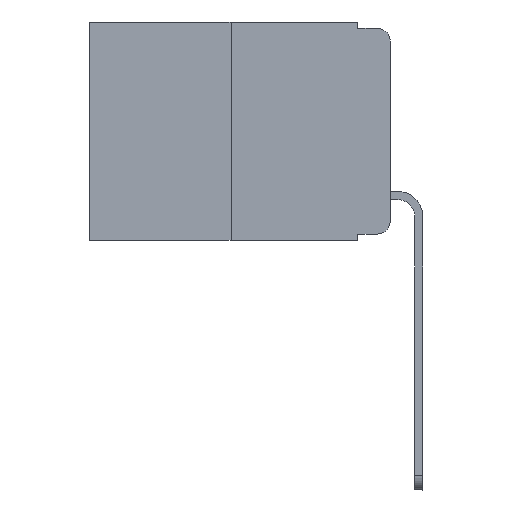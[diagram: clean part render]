
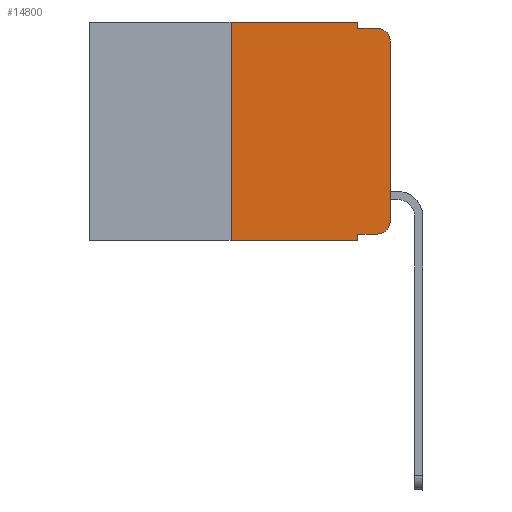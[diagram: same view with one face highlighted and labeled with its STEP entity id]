
A CAD part, left-side view. The second image highlights one B-rep face of the part: STEP entity #14800.
In plain terms, the highlighted planar face has unit normal (-1, 0, 0).
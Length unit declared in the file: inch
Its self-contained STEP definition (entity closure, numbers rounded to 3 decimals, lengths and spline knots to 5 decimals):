
#773 = EDGE_CURVE ( 'NONE', #11115, #21917, #16133, .T. ) ;
#885 = DIRECTION ( 'NONE',  ( 0., 0., 1. ) ) ;
#1099 = FACE_OUTER_BOUND ( 'NONE', #20574, .T. ) ;
#1413 = CARTESIAN_POINT ( 'NONE',  ( 0., 0., 0. ) ) ;
#1482 = CARTESIAN_POINT ( 'NONE',  ( 0., 0., -0.03 ) ) ;
#1613 = DIRECTION ( 'NONE',  ( 0., 0., -1. ) ) ;
#1844 = ORIENTED_EDGE ( 'NONE', *, *, #6821, .T. ) ;
#2396 = LINE ( 'NONE', #14699, #17212 ) ;
#2480 = VERTEX_POINT ( 'NONE', #22366 ) ;
#3273 = VECTOR ( 'NONE', #18953, 39.37008 ) ;
#3359 = EDGE_CURVE ( 'NONE', #6526, #16230, #17309, .T. ) ;
#3401 = LINE ( 'NONE', #10682, #7430 ) ;
#3406 = EDGE_CURVE ( 'NONE', #19445, #14381, #3401, .T. ) ;
#4386 = LINE ( 'NONE', #16336, #14904 ) ;
#5194 = EDGE_CURVE ( 'NONE', #18230, #22474, #4386, .T. ) ;
#5311 = CARTESIAN_POINT ( 'NONE',  ( 0., 0.051, -0.01 ) ) ;
#5613 = ORIENTED_EDGE ( 'NONE', *, *, #9055, .F. ) ;
#5789 = CARTESIAN_POINT ( 'NONE',  ( 0., 0.02, -0.03 ) ) ;
#6432 = DIRECTION ( 'NONE',  ( 0., 0., -1. ) ) ;
#6526 = VERTEX_POINT ( 'NONE', #19739 ) ;
#6821 = EDGE_CURVE ( 'NONE', #22474, #6526, #11576, .T. ) ;
#6996 = CARTESIAN_POINT ( 'NONE',  ( 0., 0.473, 0. ) ) ;
#7430 = VECTOR ( 'NONE', #21237, 39.37008 ) ;
#7449 = ORIENTED_EDGE ( 'NONE', *, *, #12989, .F. ) ;
#7861 = AXIS2_PLACEMENT_3D ( 'NONE', #15993, #15889, #1613 ) ;
#7878 = CARTESIAN_POINT ( 'NONE',  ( 0., 0.25, -0.343 ) ) ;
#7992 = CARTESIAN_POINT ( 'NONE',  ( 0., 0.02, -0.333 ) ) ;
#8171 = PLANE ( 'NONE',  #14082 ) ;
#8778 = VECTOR ( 'NONE', #12387, 39.37008 ) ;
#9055 = EDGE_CURVE ( 'NONE', #21917, #19445, #17454, .T. ) ;
#9181 = ORIENTED_EDGE ( 'NONE', *, *, #5194, .T. ) ;
#9367 = DIRECTION ( 'NONE',  ( -1., 0., 0. ) ) ;
#9678 = DIRECTION ( 'NONE',  ( 0., -1., 0. ) ) ;
#9724 = CIRCLE ( 'NONE', #22695, 0.02 ) ;
#10010 = CARTESIAN_POINT ( 'NONE',  ( 0., 0.051, -0.333 ) ) ;
#10131 = ORIENTED_EDGE ( 'NONE', *, *, #3359, .T. ) ;
#10600 = DIRECTION ( 'NONE',  ( 0., -1., 0. ) ) ;
#10682 = CARTESIAN_POINT ( 'NONE',  ( 0., 0.051, 0. ) ) ;
#11115 = VERTEX_POINT ( 'NONE', #7878 ) ;
#11576 = CIRCLE ( 'NONE', #7861, 0.02 ) ;
#11868 = CARTESIAN_POINT ( 'NONE',  ( 0., 0.051, 0. ) ) ;
#11870 = VECTOR ( 'NONE', #22622, 39.37008 ) ;
#12238 = CARTESIAN_POINT ( 'NONE',  ( 0., 0.051, 0. ) ) ;
#12387 = DIRECTION ( 'NONE',  ( 0., -1., 0. ) ) ;
#12637 = CARTESIAN_POINT ( 'NONE',  ( 0., 0.051, -0.01 ) ) ;
#12989 = EDGE_CURVE ( 'NONE', #14381, #2480, #21189, .T. ) ;
#13063 = ORIENTED_EDGE ( 'NONE', *, *, #22277, .F. ) ;
#13073 = CARTESIAN_POINT ( 'NONE',  ( 0., 0.25, 0. ) ) ;
#13086 = CARTESIAN_POINT ( 'NONE',  ( 0., 0.051, -0.343 ) ) ;
#13557 = ORIENTED_EDGE ( 'NONE', *, *, #16058, .T. ) ;
#13902 = VECTOR ( 'NONE', #885, 39.37008 ) ;
#14082 = AXIS2_PLACEMENT_3D ( 'NONE', #15252, #22323, #6432 ) ;
#14381 = VERTEX_POINT ( 'NONE', #12637 ) ;
#14699 = CARTESIAN_POINT ( 'NONE',  ( 0., 0.473, -0.343 ) ) ;
#14800 = ADVANCED_FACE ( 'NONE', ( #1099 ), #8171, .F. ) ;
#14904 = VECTOR ( 'NONE', #20279, 39.37008 ) ;
#15156 = ORIENTED_EDGE ( 'NONE', *, *, #773, .F. ) ;
#15252 = CARTESIAN_POINT ( 'NONE',  ( 0., 0.473, 0. ) ) ;
#15889 = DIRECTION ( 'NONE',  ( -1., 0., 0. ) ) ;
#15993 = CARTESIAN_POINT ( 'NONE',  ( 0., 0.02, -0.313 ) ) ;
#16058 = EDGE_CURVE ( 'NONE', #16230, #2480, #9724, .T. ) ;
#16133 = LINE ( 'NONE', #13073, #13902 ) ;
#16230 = VERTEX_POINT ( 'NONE', #1482 ) ;
#16336 = CARTESIAN_POINT ( 'NONE',  ( 0., 0.051, -0.333 ) ) ;
#17095 = ORIENTED_EDGE ( 'NONE', *, *, #3406, .F. ) ;
#17212 = VECTOR ( 'NONE', #9678, 39.37008 ) ;
#17309 = LINE ( 'NONE', #1413, #11870 ) ;
#17454 = LINE ( 'NONE', #6996, #18328 ) ;
#17678 = EDGE_CURVE ( 'NONE', #11115, #21793, #2396, .T. ) ;
#18230 = VERTEX_POINT ( 'NONE', #10010 ) ;
#18328 = VECTOR ( 'NONE', #10600, 39.37008 ) ;
#18953 = DIRECTION ( 'NONE',  ( 0., 0., -1. ) ) ;
#19308 = ORIENTED_EDGE ( 'NONE', *, *, #17678, .T. ) ;
#19445 = VERTEX_POINT ( 'NONE', #12238 ) ;
#19739 = CARTESIAN_POINT ( 'NONE',  ( 0., 0., -0.313 ) ) ;
#19958 = DIRECTION ( 'NONE',  ( 0., 0., -1. ) ) ;
#20279 = DIRECTION ( 'NONE',  ( 0., -1., 0. ) ) ;
#20574 = EDGE_LOOP ( 'NONE', ( #10131, #13557, #7449, #17095, #5613, #15156, #19308, #13063, #9181, #1844 ) ) ;
#20681 = LINE ( 'NONE', #11868, #3273 ) ;
#21189 = LINE ( 'NONE', #5311, #8778 ) ;
#21237 = DIRECTION ( 'NONE',  ( 0., 0., -1. ) ) ;
#21793 = VERTEX_POINT ( 'NONE', #13086 ) ;
#21917 = VERTEX_POINT ( 'NONE', #22811 ) ;
#22277 = EDGE_CURVE ( 'NONE', #18230, #21793, #20681, .T. ) ;
#22323 = DIRECTION ( 'NONE',  ( 1., 0., 0. ) ) ;
#22366 = CARTESIAN_POINT ( 'NONE',  ( 0., 0.02, -0.01 ) ) ;
#22474 = VERTEX_POINT ( 'NONE', #7992 ) ;
#22622 = DIRECTION ( 'NONE',  ( 0., 0., 1. ) ) ;
#22695 = AXIS2_PLACEMENT_3D ( 'NONE', #5789, #9367, #19958 ) ;
#22811 = CARTESIAN_POINT ( 'NONE',  ( 0., 0.25, 0. ) ) ;
